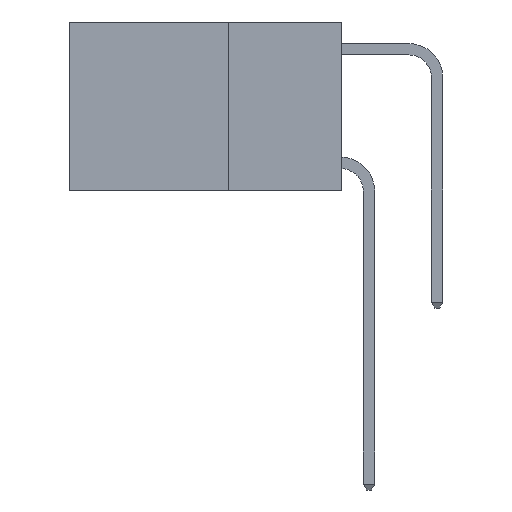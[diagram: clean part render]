
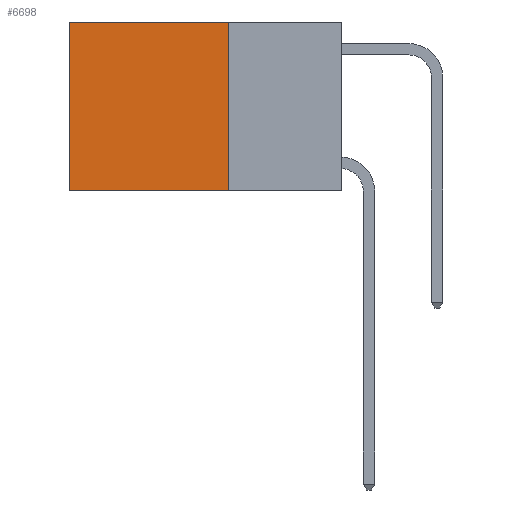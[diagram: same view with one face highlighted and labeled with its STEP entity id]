
A CAD part, left-side view. The second image highlights one B-rep face of the part: STEP entity #6698.
In plain terms, the highlighted planar face has unit normal (-1, 0, 0).
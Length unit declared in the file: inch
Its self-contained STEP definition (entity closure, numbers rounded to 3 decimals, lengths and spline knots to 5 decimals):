
#63 = ORIENTED_EDGE ( 'NONE', *, *, #8711, .T. ) ;
#649 = DIRECTION ( 'NONE',  ( 0., 0., -1. ) ) ;
#1145 = CARTESIAN_POINT ( 'NONE',  ( 0.2625, 0.25, -0.37 ) ) ;
#1152 = EDGE_CURVE ( 'NONE', #4332, #12557, #12369, .T. ) ;
#1325 = VECTOR ( 'NONE', #11524, 39.37008 ) ;
#1610 = ORIENTED_EDGE ( 'NONE', *, *, #1152, .T. ) ;
#1669 = LINE ( 'NONE', #6372, #1325 ) ;
#2148 = VERTEX_POINT ( 'NONE', #1145 ) ;
#3761 = CARTESIAN_POINT ( 'NONE',  ( 0.2625, 0.25, 0. ) ) ;
#4332 = VERTEX_POINT ( 'NONE', #12689 ) ;
#4574 = VECTOR ( 'NONE', #9865, 39.37008 ) ;
#4637 = CARTESIAN_POINT ( 'NONE',  ( 0.2625, 0.6, -0.37 ) ) ;
#5040 = VERTEX_POINT ( 'NONE', #4637 ) ;
#5532 = LINE ( 'NONE', #13367, #8617 ) ;
#5791 = AXIS2_PLACEMENT_3D ( 'NONE', #11093, #6998, #649 ) ;
#6372 = CARTESIAN_POINT ( 'NONE',  ( 0.2625, 0.25, -0.37 ) ) ;
#6698 = ADVANCED_FACE ( 'NONE', ( #10749 ), #13155, .F. ) ;
#6998 = DIRECTION ( 'NONE',  ( 1., 0., 0. ) ) ;
#8190 = ORIENTED_EDGE ( 'NONE', *, *, #10604, .F. ) ;
#8617 = VECTOR ( 'NONE', #9279, 39.37008 ) ;
#8618 = ORIENTED_EDGE ( 'NONE', *, *, #11486, .F. ) ;
#8711 = EDGE_CURVE ( 'NONE', #12557, #5040, #5532, .T. ) ;
#9279 = DIRECTION ( 'NONE',  ( 0., 0., -1. ) ) ;
#9308 = VECTOR ( 'NONE', #9965, 39.37008 ) ;
#9497 = CARTESIAN_POINT ( 'NONE',  ( 0.2625, 0.6, 0. ) ) ;
#9865 = DIRECTION ( 'NONE',  ( 0., 0., -1. ) ) ;
#9965 = DIRECTION ( 'NONE',  ( 0., 1., 0. ) ) ;
#10064 = LINE ( 'NONE', #12941, #4574 ) ;
#10604 = EDGE_CURVE ( 'NONE', #2148, #5040, #1669, .T. ) ;
#10749 = FACE_OUTER_BOUND ( 'NONE', #11889, .T. ) ;
#11093 = CARTESIAN_POINT ( 'NONE',  ( 0.2625, 0.25, 0. ) ) ;
#11486 = EDGE_CURVE ( 'NONE', #4332, #2148, #10064, .T. ) ;
#11524 = DIRECTION ( 'NONE',  ( 0., 1., 0. ) ) ;
#11889 = EDGE_LOOP ( 'NONE', ( #63, #8190, #8618, #1610 ) ) ;
#12369 = LINE ( 'NONE', #3761, #9308 ) ;
#12557 = VERTEX_POINT ( 'NONE', #9497 ) ;
#12689 = CARTESIAN_POINT ( 'NONE',  ( 0.2625, 0.25, 0. ) ) ;
#12941 = CARTESIAN_POINT ( 'NONE',  ( 0.2625, 0.25, 0. ) ) ;
#13155 = PLANE ( 'NONE',  #5791 ) ;
#13367 = CARTESIAN_POINT ( 'NONE',  ( 0.2625, 0.6, 0. ) ) ;
